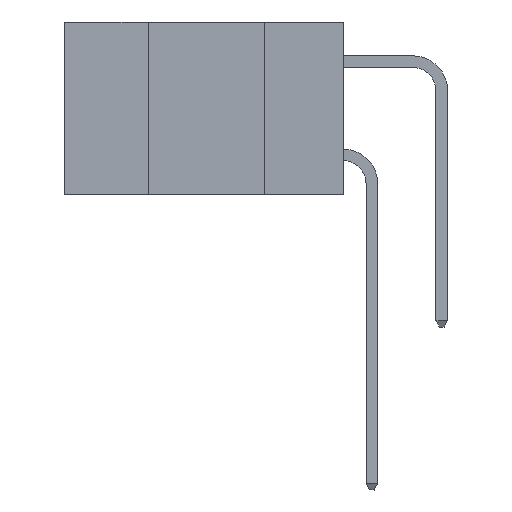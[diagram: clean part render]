
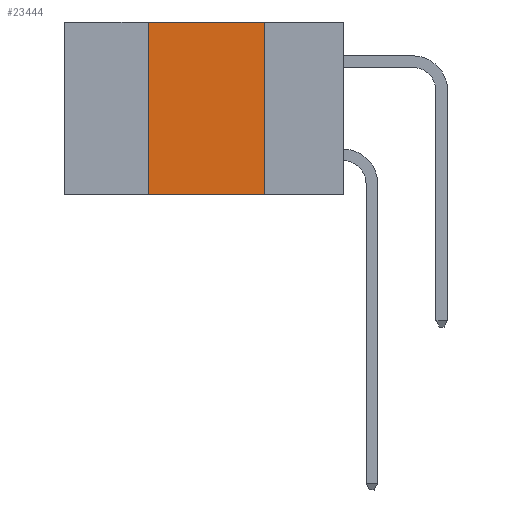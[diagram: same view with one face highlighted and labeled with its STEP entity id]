
A CAD part, left-side view. The second image highlights one B-rep face of the part: STEP entity #23444.
In plain terms, the highlighted planar face has unit normal (-1, 0, 0).
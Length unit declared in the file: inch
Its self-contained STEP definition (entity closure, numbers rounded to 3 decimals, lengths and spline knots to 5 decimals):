
#121 = LINE ( 'NONE', #12347, #19001 ) ;
#1132 = DIRECTION ( 'NONE',  ( 0., 0., -1. ) ) ;
#1137 = CARTESIAN_POINT ( 'NONE',  ( 0., 0.42, 0. ) ) ;
#1495 = VERTEX_POINT ( 'NONE', #12669 ) ;
#2758 = DIRECTION ( 'NONE',  ( 0., 0., 1. ) ) ;
#3057 = CARTESIAN_POINT ( 'NONE',  ( 0., 0.6, 0. ) ) ;
#3126 = VERTEX_POINT ( 'NONE', #23063 ) ;
#3510 = EDGE_LOOP ( 'NONE', ( #12808, #20448, #23761, #10275 ) ) ;
#3604 = EDGE_CURVE ( 'NONE', #12591, #1495, #121, .T. ) ;
#4904 = EDGE_CURVE ( 'NONE', #24816, #12591, #8277, .T. ) ;
#5201 = AXIS2_PLACEMENT_3D ( 'NONE', #3057, #23919, #1132 ) ;
#6514 = CARTESIAN_POINT ( 'NONE',  ( 0., 0.17, 0. ) ) ;
#8277 = LINE ( 'NONE', #22582, #15871 ) ;
#8305 = DIRECTION ( 'NONE',  ( 0., -1., 0. ) ) ;
#10275 = ORIENTED_EDGE ( 'NONE', *, *, #13882, .T. ) ;
#11301 = PLANE ( 'NONE',  #5201 ) ;
#12347 = CARTESIAN_POINT ( 'NONE',  ( 0., 0.17, -0.37 ) ) ;
#12591 = VERTEX_POINT ( 'NONE', #6514 ) ;
#12669 = CARTESIAN_POINT ( 'NONE',  ( 0., 0.17, -0.37 ) ) ;
#12808 = ORIENTED_EDGE ( 'NONE', *, *, #3604, .F. ) ;
#12919 = LINE ( 'NONE', #23348, #24098 ) ;
#13882 = EDGE_CURVE ( 'NONE', #3126, #1495, #14362, .T. ) ;
#14362 = LINE ( 'NONE', #22736, #24446 ) ;
#15555 = FACE_OUTER_BOUND ( 'NONE', #3510, .T. ) ;
#15871 = VECTOR ( 'NONE', #18215, 39.37008 ) ;
#18215 = DIRECTION ( 'NONE',  ( 0., -1., 0. ) ) ;
#18807 = DIRECTION ( 'NONE',  ( 0., 0., -1. ) ) ;
#19001 = VECTOR ( 'NONE', #18807, 39.37008 ) ;
#20448 = ORIENTED_EDGE ( 'NONE', *, *, #4904, .F. ) ;
#22582 = CARTESIAN_POINT ( 'NONE',  ( 0., 0.6, 0. ) ) ;
#22736 = CARTESIAN_POINT ( 'NONE',  ( 0., 0.6, -0.37 ) ) ;
#23063 = CARTESIAN_POINT ( 'NONE',  ( 0., 0.42, -0.37 ) ) ;
#23348 = CARTESIAN_POINT ( 'NONE',  ( 0., 0.42, -0.37 ) ) ;
#23444 = ADVANCED_FACE ( 'NONE', ( #15555 ), #11301, .F. ) ;
#23761 = ORIENTED_EDGE ( 'NONE', *, *, #26667, .F. ) ;
#23919 = DIRECTION ( 'NONE',  ( 1., 0., 0. ) ) ;
#24098 = VECTOR ( 'NONE', #2758, 39.37008 ) ;
#24446 = VECTOR ( 'NONE', #8305, 39.37008 ) ;
#24816 = VERTEX_POINT ( 'NONE', #1137 ) ;
#26667 = EDGE_CURVE ( 'NONE', #3126, #24816, #12919, .T. ) ;
